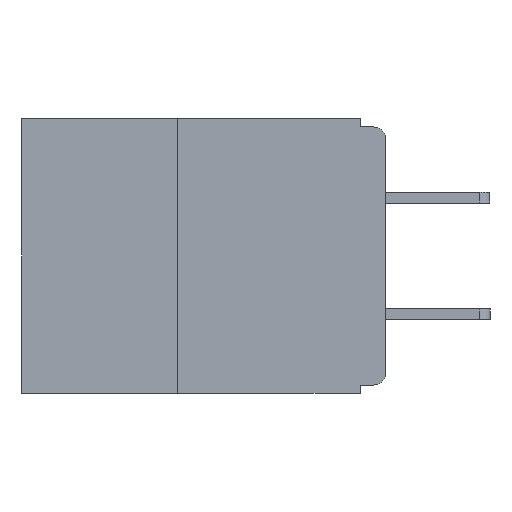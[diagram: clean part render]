
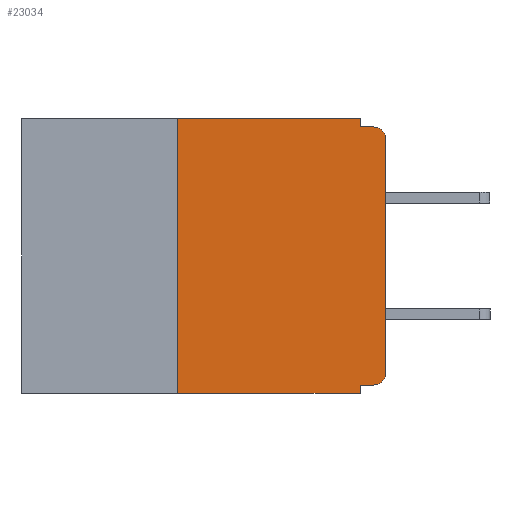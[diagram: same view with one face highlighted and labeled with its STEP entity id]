
A CAD part, left-side view. The second image highlights one B-rep face of the part: STEP entity #23034.
In plain terms, the highlighted planar face has unit normal (-1, 0, 0).
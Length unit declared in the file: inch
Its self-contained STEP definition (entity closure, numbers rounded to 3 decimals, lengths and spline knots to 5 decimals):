
#27 = VECTOR ( 'NONE', #16659, 39.37008 ) ;
#232 = ORIENTED_EDGE ( 'NONE', *, *, #22890, .F. ) ;
#993 = EDGE_CURVE ( 'NONE', #9481, #8684, #10188, .T. ) ;
#1696 = CARTESIAN_POINT ( 'NONE',  ( 0., 0.437, -0.33 ) ) ;
#2200 = CARTESIAN_POINT ( 'NONE',  ( 0., 0.031, 0. ) ) ;
#2378 = VECTOR ( 'NONE', #20850, 39.37008 ) ;
#2565 = ORIENTED_EDGE ( 'NONE', *, *, #21856, .T. ) ;
#2577 = ORIENTED_EDGE ( 'NONE', *, *, #3247, .F. ) ;
#2694 = CARTESIAN_POINT ( 'NONE',  ( 0., 0.015, -0.025 ) ) ;
#2989 = LINE ( 'NONE', #2200, #2378 ) ;
#3058 = VERTEX_POINT ( 'NONE', #19097 ) ;
#3228 = VERTEX_POINT ( 'NONE', #17073 ) ;
#3247 = EDGE_CURVE ( 'NONE', #4655, #15982, #5713, .T. ) ;
#3323 = DIRECTION ( 'NONE',  ( 0., 0., -1. ) ) ;
#3370 = DIRECTION ( 'NONE',  ( -1., 0., 0. ) ) ;
#3914 = EDGE_LOOP ( 'NONE', ( #2565, #17978, #22566, #232, #5000, #5827, #12545, #17095, #2577, #18315 ) ) ;
#4304 = AXIS2_PLACEMENT_3D ( 'NONE', #2694, #15743, #4607 ) ;
#4607 = DIRECTION ( 'NONE',  ( 0., 0., -1. ) ) ;
#4655 = VERTEX_POINT ( 'NONE', #9355 ) ;
#4985 = VERTEX_POINT ( 'NONE', #21914 ) ;
#5000 = ORIENTED_EDGE ( 'NONE', *, *, #993, .F. ) ;
#5205 = CARTESIAN_POINT ( 'NONE',  ( 0., 0., -0.025 ) ) ;
#5713 = LINE ( 'NONE', #16992, #27 ) ;
#5827 = ORIENTED_EDGE ( 'NONE', *, *, #21681, .F. ) ;
#6001 = VECTOR ( 'NONE', #22898, 39.37008 ) ;
#6338 = CARTESIAN_POINT ( 'NONE',  ( 0., 0.25, -0.33 ) ) ;
#6440 = CARTESIAN_POINT ( 'NONE',  ( 0., 0.437, 0. ) ) ;
#6812 = CARTESIAN_POINT ( 'NONE',  ( 0., 0., 0. ) ) ;
#7129 = CARTESIAN_POINT ( 'NONE',  ( 0., 0.031, -0.33 ) ) ;
#7462 = VECTOR ( 'NONE', #8708, 39.37008 ) ;
#8409 = PLANE ( 'NONE',  #21364 ) ;
#8450 = AXIS2_PLACEMENT_3D ( 'NONE', #14555, #3370, #16377 ) ;
#8684 = VERTEX_POINT ( 'NONE', #15642 ) ;
#8708 = DIRECTION ( 'NONE',  ( 0., 0., 1. ) ) ;
#9051 = DIRECTION ( 'NONE',  ( 0., -1., 0. ) ) ;
#9355 = CARTESIAN_POINT ( 'NONE',  ( 0., 0.015, -0.32 ) ) ;
#9481 = VERTEX_POINT ( 'NONE', #12353 ) ;
#10188 = LINE ( 'NONE', #10381, #18778 ) ;
#10263 = DIRECTION ( 'NONE',  ( 0., 0., -1. ) ) ;
#10381 = CARTESIAN_POINT ( 'NONE',  ( 0., 0.437, 0. ) ) ;
#10891 = CARTESIAN_POINT ( 'NONE',  ( 0., 0.031, -0.32 ) ) ;
#10953 = LINE ( 'NONE', #6338, #6001 ) ;
#11026 = DIRECTION ( 'NONE',  ( 0., -1., 0. ) ) ;
#12177 = VECTOR ( 'NONE', #3323, 39.37008 ) ;
#12353 = CARTESIAN_POINT ( 'NONE',  ( 0., 0.25, 0. ) ) ;
#12422 = CIRCLE ( 'NONE', #8450, 0.015 ) ;
#12545 = ORIENTED_EDGE ( 'NONE', *, *, #20440, .T. ) ;
#13296 = EDGE_CURVE ( 'NONE', #4985, #17828, #18393, .T. ) ;
#13630 = VECTOR ( 'NONE', #14811, 39.37008 ) ;
#14387 = FACE_OUTER_BOUND ( 'NONE', #3914, .T. ) ;
#14555 = CARTESIAN_POINT ( 'NONE',  ( 0., 0.015, -0.305 ) ) ;
#14811 = DIRECTION ( 'NONE',  ( 0., -1., 0. ) ) ;
#15642 = CARTESIAN_POINT ( 'NONE',  ( 0., 0.031, 0. ) ) ;
#15743 = DIRECTION ( 'NONE',  ( -1., 0., 0. ) ) ;
#15982 = VERTEX_POINT ( 'NONE', #10891 ) ;
#16377 = DIRECTION ( 'NONE',  ( 0., 0., -1. ) ) ;
#16454 = CARTESIAN_POINT ( 'NONE',  ( 0., 0., -0.01 ) ) ;
#16519 = CARTESIAN_POINT ( 'NONE',  ( 0., 0.015, -0.01 ) ) ;
#16659 = DIRECTION ( 'NONE',  ( 0., 1., 0. ) ) ;
#16992 = CARTESIAN_POINT ( 'NONE',  ( 0., 0., -0.32 ) ) ;
#17073 = CARTESIAN_POINT ( 'NONE',  ( 0., 0.031, -0.33 ) ) ;
#17095 = ORIENTED_EDGE ( 'NONE', *, *, #17980, .F. ) ;
#17135 = VERTEX_POINT ( 'NONE', #17895 ) ;
#17828 = VERTEX_POINT ( 'NONE', #16519 ) ;
#17895 = CARTESIAN_POINT ( 'NONE',  ( 0., 0.25, -0.33 ) ) ;
#17978 = ORIENTED_EDGE ( 'NONE', *, *, #21075, .T. ) ;
#17980 = EDGE_CURVE ( 'NONE', #15982, #3228, #21880, .T. ) ;
#18315 = ORIENTED_EDGE ( 'NONE', *, *, #18603, .T. ) ;
#18393 = LINE ( 'NONE', #16454, #22682 ) ;
#18465 = LINE ( 'NONE', #1696, #13630 ) ;
#18603 = EDGE_CURVE ( 'NONE', #4655, #3058, #12422, .T. ) ;
#18778 = VECTOR ( 'NONE', #11026, 39.37008 ) ;
#19097 = CARTESIAN_POINT ( 'NONE',  ( 0., 0., -0.305 ) ) ;
#19277 = CIRCLE ( 'NONE', #4304, 0.015 ) ;
#20396 = VERTEX_POINT ( 'NONE', #5205 ) ;
#20440 = EDGE_CURVE ( 'NONE', #17135, #3228, #18465, .T. ) ;
#20850 = DIRECTION ( 'NONE',  ( 0., 0., -1. ) ) ;
#21075 = EDGE_CURVE ( 'NONE', #20396, #17828, #19277, .T. ) ;
#21250 = DIRECTION ( 'NONE',  ( 1., 0., 0. ) ) ;
#21364 = AXIS2_PLACEMENT_3D ( 'NONE', #6440, #21250, #10263 ) ;
#21681 = EDGE_CURVE ( 'NONE', #17135, #9481, #10953, .T. ) ;
#21856 = EDGE_CURVE ( 'NONE', #3058, #20396, #22115, .T. ) ;
#21880 = LINE ( 'NONE', #7129, #12177 ) ;
#21914 = CARTESIAN_POINT ( 'NONE',  ( 0., 0.031, -0.01 ) ) ;
#22115 = LINE ( 'NONE', #6812, #7462 ) ;
#22566 = ORIENTED_EDGE ( 'NONE', *, *, #13296, .F. ) ;
#22682 = VECTOR ( 'NONE', #9051, 39.37008 ) ;
#22890 = EDGE_CURVE ( 'NONE', #8684, #4985, #2989, .T. ) ;
#22898 = DIRECTION ( 'NONE',  ( 0., 0., 1. ) ) ;
#23034 = ADVANCED_FACE ( 'NONE', ( #14387 ), #8409, .F. ) ;
